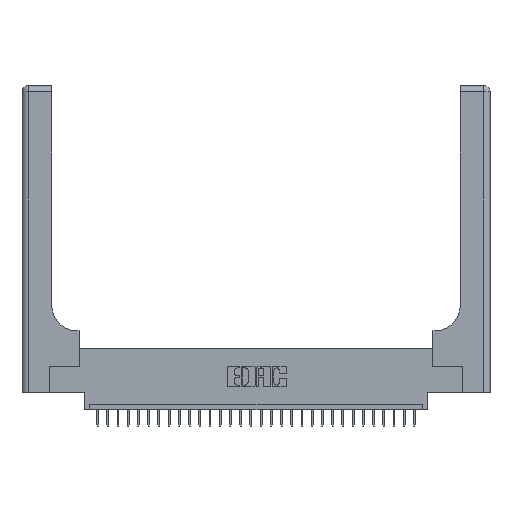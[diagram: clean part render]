
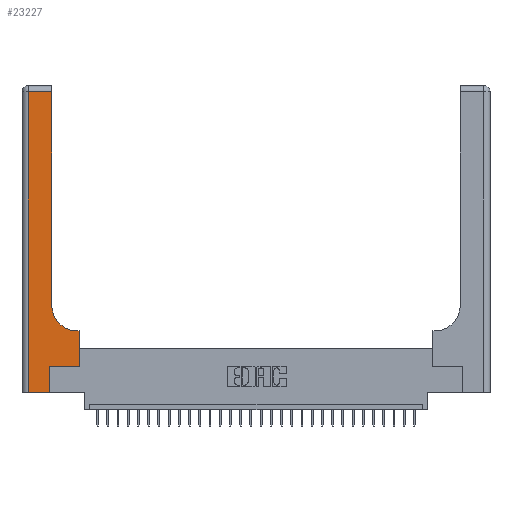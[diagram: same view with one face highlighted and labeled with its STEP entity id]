
A CAD part, top view. The second image highlights one B-rep face of the part: STEP entity #23227.
In plain terms, the highlighted planar face has unit normal (0, 0, 1).
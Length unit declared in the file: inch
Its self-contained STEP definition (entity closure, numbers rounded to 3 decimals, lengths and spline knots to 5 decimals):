
#170 = VECTOR ( 'NONE', #24291, 39.37008 ) ;
#212 = AXIS2_PLACEMENT_3D ( 'NONE', #19496, #24262, #10038 ) ;
#1046 = CARTESIAN_POINT ( 'NONE',  ( 0.269, 0.25, 0.37 ) ) ;
#1196 = CIRCLE ( 'NONE', #14109, 0.25 ) ;
#1442 = VECTOR ( 'NONE', #28538, 39.37008 ) ;
#1705 = DIRECTION ( 'NONE',  ( -1., 0., 0. ) ) ;
#2197 = VERTEX_POINT ( 'NONE', #2835 ) ;
#2787 = LINE ( 'NONE', #8506, #6074 ) ;
#2835 = CARTESIAN_POINT ( 'NONE',  ( 0.5585, 0.6, 0.37 ) ) ;
#3491 = ORIENTED_EDGE ( 'NONE', *, *, #27810, .T. ) ;
#3962 = VECTOR ( 'NONE', #20377, 39.37008 ) ;
#4713 = EDGE_CURVE ( 'NONE', #25529, #29466, #2787, .T. ) ;
#5279 = CARTESIAN_POINT ( 'NONE',  ( 0.269, 0.25, 0.37 ) ) ;
#5695 = CARTESIAN_POINT ( 'NONE',  ( 0.5415, 0.6, 0.37 ) ) ;
#5958 = EDGE_CURVE ( 'NONE', #24404, #10407, #1196, .T. ) ;
#6074 = VECTOR ( 'NONE', #22829, 39.37008 ) ;
#6387 = VECTOR ( 'NONE', #1705, 39.37008 ) ;
#7351 = DIRECTION ( 'NONE',  ( -1., 0., 0. ) ) ;
#7445 = VERTEX_POINT ( 'NONE', #21336 ) ;
#8506 = CARTESIAN_POINT ( 'NONE',  ( 0.06, 3., 0.37 ) ) ;
#8740 = CARTESIAN_POINT ( 'NONE',  ( 0.269, 0., 0.37 ) ) ;
#9489 = CARTESIAN_POINT ( 'NONE',  ( 0.269, 0., 0.37 ) ) ;
#9610 = CARTESIAN_POINT ( 'NONE',  ( 0.2915, 3., 0.37 ) ) ;
#9799 = EDGE_CURVE ( 'NONE', #7445, #2197, #19157, .T. ) ;
#10038 = DIRECTION ( 'NONE',  ( -1., 0., 0. ) ) ;
#10137 = ORIENTED_EDGE ( 'NONE', *, *, #28859, .T. ) ;
#10145 = EDGE_CURVE ( 'NONE', #28219, #7445, #27380, .T. ) ;
#10269 = LINE ( 'NONE', #8740, #3962 ) ;
#10407 = VERTEX_POINT ( 'NONE', #24093 ) ;
#10744 = ORIENTED_EDGE ( 'NONE', *, *, #4713, .T. ) ;
#10968 = CARTESIAN_POINT ( 'NONE',  ( 0.5415, 0.85, 0.37 ) ) ;
#11172 = DIRECTION ( 'NONE',  ( 1., 0., 0. ) ) ;
#11232 = LINE ( 'NONE', #9610, #24257 ) ;
#11356 = EDGE_CURVE ( 'NONE', #2197, #24404, #26894, .T. ) ;
#11884 = VERTEX_POINT ( 'NONE', #14475 ) ;
#12820 = PLANE ( 'NONE',  #212 ) ;
#14109 = AXIS2_PLACEMENT_3D ( 'NONE', #10968, #30002, #11172 ) ;
#14245 = DIRECTION ( 'NONE',  ( 0., 1., 0. ) ) ;
#14436 = CARTESIAN_POINT ( 'NONE',  ( 0., 0., 0.37 ) ) ;
#14475 = CARTESIAN_POINT ( 'NONE',  ( 0.2915, 2.94, 0.37 ) ) ;
#14733 = FACE_OUTER_BOUND ( 'NONE', #28889, .T. ) ;
#14908 = LINE ( 'NONE', #19304, #25339 ) ;
#15589 = ORIENTED_EDGE ( 'NONE', *, *, #23993, .T. ) ;
#15826 = ORIENTED_EDGE ( 'NONE', *, *, #30060, .T. ) ;
#16114 = ORIENTED_EDGE ( 'NONE', *, *, #10145, .T. ) ;
#18387 = VERTEX_POINT ( 'NONE', #9489 ) ;
#18433 = CARTESIAN_POINT ( 'NONE',  ( 0.2915, 0.6, 0.37 ) ) ;
#19157 = LINE ( 'NONE', #29500, #29954 ) ;
#19304 = CARTESIAN_POINT ( 'NONE',  ( 0., 2.94, 0.37 ) ) ;
#19496 = CARTESIAN_POINT ( 'NONE',  ( 0., 3., 0.37 ) ) ;
#20377 = DIRECTION ( 'NONE',  ( 0., 1., 0. ) ) ;
#20391 = LINE ( 'NONE', #14436, #1442 ) ;
#21336 = CARTESIAN_POINT ( 'NONE',  ( 0.5585, 0.25, 0.37 ) ) ;
#21450 = ORIENTED_EDGE ( 'NONE', *, *, #11356, .T. ) ;
#21755 = CARTESIAN_POINT ( 'NONE',  ( 0.06, 2.94, 0.37 ) ) ;
#22829 = DIRECTION ( 'NONE',  ( 0., -1., 0. ) ) ;
#23227 = ADVANCED_FACE ( 'NONE', ( #14733 ), #12820, .F. ) ;
#23993 = EDGE_CURVE ( 'NONE', #18387, #28219, #10269, .T. ) ;
#24080 = ORIENTED_EDGE ( 'NONE', *, *, #9799, .T. ) ;
#24093 = CARTESIAN_POINT ( 'NONE',  ( 0.2915, 0.85, 0.37 ) ) ;
#24257 = VECTOR ( 'NONE', #14245, 39.37008 ) ;
#24262 = DIRECTION ( 'NONE',  ( 0., 0., -1. ) ) ;
#24291 = DIRECTION ( 'NONE',  ( 1., 0., 0. ) ) ;
#24404 = VERTEX_POINT ( 'NONE', #5695 ) ;
#25339 = VECTOR ( 'NONE', #7351, 39.37008 ) ;
#25529 = VERTEX_POINT ( 'NONE', #21755 ) ;
#26894 = LINE ( 'NONE', #18433, #6387 ) ;
#27070 = ORIENTED_EDGE ( 'NONE', *, *, #5958, .T. ) ;
#27380 = LINE ( 'NONE', #5279, #170 ) ;
#27810 = EDGE_CURVE ( 'NONE', #10407, #11884, #11232, .T. ) ;
#28219 = VERTEX_POINT ( 'NONE', #1046 ) ;
#28538 = DIRECTION ( 'NONE',  ( 1., 0., 0. ) ) ;
#28664 = CARTESIAN_POINT ( 'NONE',  ( 0.06, 0., 0.37 ) ) ;
#28859 = EDGE_CURVE ( 'NONE', #11884, #25529, #14908, .T. ) ;
#28889 = EDGE_LOOP ( 'NONE', ( #3491, #10137, #10744, #15826, #15589, #16114, #24080, #21450, #27070 ) ) ;
#29466 = VERTEX_POINT ( 'NONE', #28664 ) ;
#29500 = CARTESIAN_POINT ( 'NONE',  ( 0.5585, 0.25, 0.37 ) ) ;
#29698 = DIRECTION ( 'NONE',  ( 0., 1., 0. ) ) ;
#29954 = VECTOR ( 'NONE', #29698, 39.37008 ) ;
#30002 = DIRECTION ( 'NONE',  ( 0., 0., -1. ) ) ;
#30060 = EDGE_CURVE ( 'NONE', #29466, #18387, #20391, .T. ) ;
